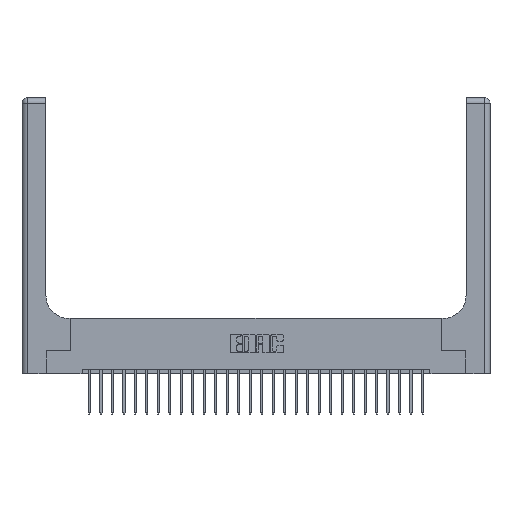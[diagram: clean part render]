
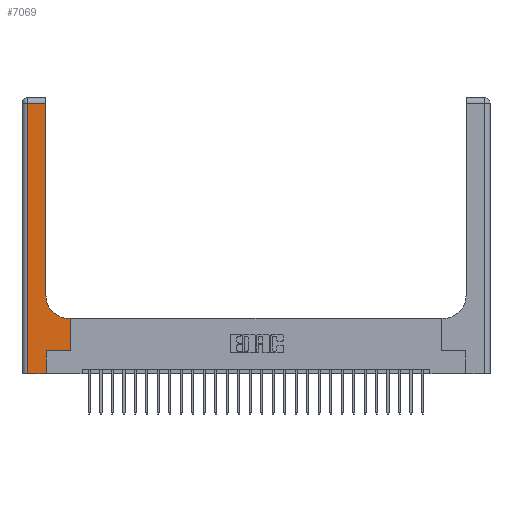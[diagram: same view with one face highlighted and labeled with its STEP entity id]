
A CAD part, top view. The second image highlights one B-rep face of the part: STEP entity #7069.
In plain terms, the highlighted planar face has unit normal (0, 0, 1).
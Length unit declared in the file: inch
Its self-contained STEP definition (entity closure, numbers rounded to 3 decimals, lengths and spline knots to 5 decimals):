
#272 = LINE ( 'NONE', #6495, #2966 ) ;
#1709 = CARTESIAN_POINT ( 'NONE',  ( 0.265, 0., 0.37 ) ) ;
#2579 = VERTEX_POINT ( 'NONE', #6363 ) ;
#2966 = VECTOR ( 'NONE', #12450, 39.37008 ) ;
#3351 = CARTESIAN_POINT ( 'NONE',  ( 0.06, 0., 0.37 ) ) ;
#3836 = VERTEX_POINT ( 'NONE', #16934 ) ;
#3861 = CARTESIAN_POINT ( 'NONE',  ( 0.26, 0.85, 0.37 ) ) ;
#3908 = CARTESIAN_POINT ( 'NONE',  ( 0.265, 0.25, 0.37 ) ) ;
#3955 = CARTESIAN_POINT ( 'NONE',  ( 0.06, 2.94, 0.37 ) ) ;
#4228 = EDGE_CURVE ( 'NONE', #3836, #20699, #10779, .T. ) ;
#4561 = VECTOR ( 'NONE', #22025, 39.37008 ) ;
#4711 = FACE_OUTER_BOUND ( 'NONE', #15910, .T. ) ;
#5549 = CARTESIAN_POINT ( 'NONE',  ( 0.265, 0.25, 0.37 ) ) ;
#5748 = VERTEX_POINT ( 'NONE', #3955 ) ;
#5836 = VECTOR ( 'NONE', #26196, 39.37008 ) ;
#6363 = CARTESIAN_POINT ( 'NONE',  ( 0.265, 0., 0.37 ) ) ;
#6495 = CARTESIAN_POINT ( 'NONE',  ( 0., 0., 0.37 ) ) ;
#6656 = DIRECTION ( 'NONE',  ( 0., 0., -1. ) ) ;
#6881 = PLANE ( 'NONE',  #18829 ) ;
#6960 = VERTEX_POINT ( 'NONE', #3351 ) ;
#6987 = CARTESIAN_POINT ( 'NONE',  ( 0.26, 2.94, 0.37 ) ) ;
#7069 = ADVANCED_FACE ( 'NONE', ( #4711 ), #6881, .F. ) ;
#7849 = EDGE_CURVE ( 'NONE', #5748, #6960, #18246, .T. ) ;
#8076 = VECTOR ( 'NONE', #26592, 39.37008 ) ;
#8552 = ORIENTED_EDGE ( 'NONE', *, *, #22328, .T. ) ;
#9588 = CARTESIAN_POINT ( 'NONE',  ( 0.26, 0.6, 0.37 ) ) ;
#10045 = VERTEX_POINT ( 'NONE', #14085 ) ;
#10185 = EDGE_CURVE ( 'NONE', #6960, #2579, #272, .T. ) ;
#10580 = EDGE_CURVE ( 'NONE', #20699, #10045, #20230, .T. ) ;
#10625 = ORIENTED_EDGE ( 'NONE', *, *, #18327, .T. ) ;
#10779 = LINE ( 'NONE', #25227, #23381 ) ;
#11319 = CARTESIAN_POINT ( 'NONE',  ( 0.26, 3., 0.37 ) ) ;
#11390 = LINE ( 'NONE', #5549, #4561 ) ;
#11597 = CARTESIAN_POINT ( 'NONE',  ( 0., 2.94, 0.37 ) ) ;
#11876 = DIRECTION ( 'NONE',  ( -1., 0., 0. ) ) ;
#12012 = LINE ( 'NONE', #1709, #8076 ) ;
#12116 = VERTEX_POINT ( 'NONE', #6987 ) ;
#12146 = CIRCLE ( 'NONE', #20442, 0.25 ) ;
#12450 = DIRECTION ( 'NONE',  ( 1., 0., 0. ) ) ;
#12516 = CARTESIAN_POINT ( 'NONE',  ( 0.528, 0.6, 0.37 ) ) ;
#12619 = CARTESIAN_POINT ( 'NONE',  ( 0.51, 0.85, 0.37 ) ) ;
#12688 = ORIENTED_EDGE ( 'NONE', *, *, #15168, .T. ) ;
#12810 = DIRECTION ( 'NONE',  ( 0., 1., 0. ) ) ;
#13068 = VECTOR ( 'NONE', #11876, 39.37008 ) ;
#14085 = CARTESIAN_POINT ( 'NONE',  ( 0.51, 0.6, 0.37 ) ) ;
#14595 = VERTEX_POINT ( 'NONE', #3908 ) ;
#14627 = DIRECTION ( 'NONE',  ( -1., 0., 0. ) ) ;
#15168 = EDGE_CURVE ( 'NONE', #2579, #14595, #12012, .T. ) ;
#15270 = ORIENTED_EDGE ( 'NONE', *, *, #4228, .T. ) ;
#15539 = LINE ( 'NONE', #11319, #19319 ) ;
#15910 = EDGE_LOOP ( 'NONE', ( #10625, #19808, #25275, #19757, #12688, #22172, #15270, #19179, #8552 ) ) ;
#16934 = CARTESIAN_POINT ( 'NONE',  ( 0.528, 0.25, 0.37 ) ) ;
#18246 = LINE ( 'NONE', #18381, #21568 ) ;
#18327 = EDGE_CURVE ( 'NONE', #25196, #12116, #15539, .T. ) ;
#18381 = CARTESIAN_POINT ( 'NONE',  ( 0.06, 3., 0.37 ) ) ;
#18829 = AXIS2_PLACEMENT_3D ( 'NONE', #23243, #25132, #14627 ) ;
#18841 = EDGE_CURVE ( 'NONE', #14595, #3836, #11390, .T. ) ;
#19179 = ORIENTED_EDGE ( 'NONE', *, *, #10580, .T. ) ;
#19319 = VECTOR ( 'NONE', #19644, 39.37008 ) ;
#19644 = DIRECTION ( 'NONE',  ( 0., 1., 0. ) ) ;
#19757 = ORIENTED_EDGE ( 'NONE', *, *, #10185, .T. ) ;
#19808 = ORIENTED_EDGE ( 'NONE', *, *, #23973, .T. ) ;
#20230 = LINE ( 'NONE', #9588, #5836 ) ;
#20442 = AXIS2_PLACEMENT_3D ( 'NONE', #12619, #6656, #23139 ) ;
#20699 = VERTEX_POINT ( 'NONE', #12516 ) ;
#21568 = VECTOR ( 'NONE', #22481, 39.37008 ) ;
#22025 = DIRECTION ( 'NONE',  ( 1., 0., 0. ) ) ;
#22172 = ORIENTED_EDGE ( 'NONE', *, *, #18841, .T. ) ;
#22328 = EDGE_CURVE ( 'NONE', #10045, #25196, #12146, .T. ) ;
#22481 = DIRECTION ( 'NONE',  ( 0., -1., 0. ) ) ;
#23139 = DIRECTION ( 'NONE',  ( 1., 0., 0. ) ) ;
#23243 = CARTESIAN_POINT ( 'NONE',  ( 0., 3., 0.37 ) ) ;
#23381 = VECTOR ( 'NONE', #12810, 39.37008 ) ;
#23973 = EDGE_CURVE ( 'NONE', #12116, #5748, #24543, .T. ) ;
#24543 = LINE ( 'NONE', #11597, #13068 ) ;
#25132 = DIRECTION ( 'NONE',  ( 0., 0., -1. ) ) ;
#25196 = VERTEX_POINT ( 'NONE', #3861 ) ;
#25227 = CARTESIAN_POINT ( 'NONE',  ( 0.528, 0.25, 0.37 ) ) ;
#25275 = ORIENTED_EDGE ( 'NONE', *, *, #7849, .T. ) ;
#26196 = DIRECTION ( 'NONE',  ( -1., 0., 0. ) ) ;
#26592 = DIRECTION ( 'NONE',  ( 0., 1., 0. ) ) ;
